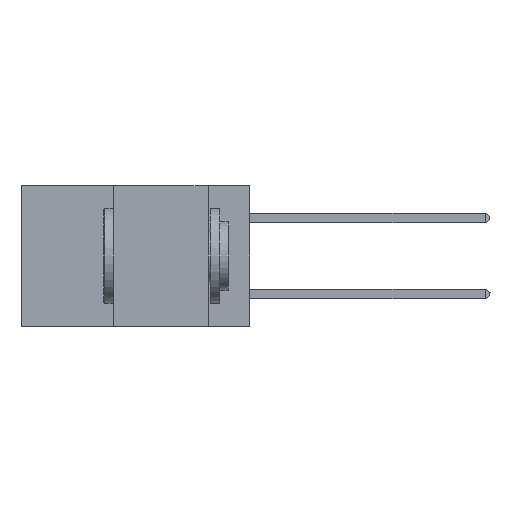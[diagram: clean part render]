
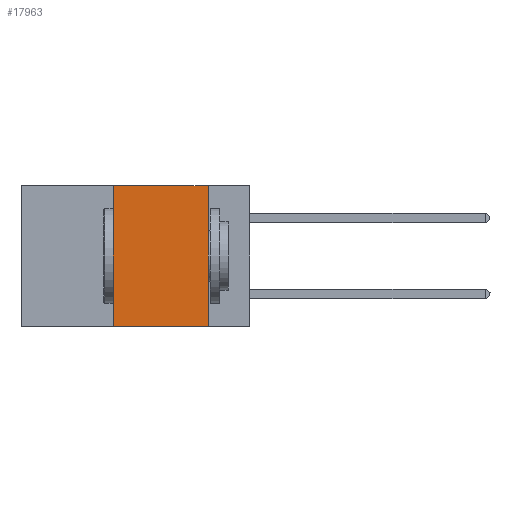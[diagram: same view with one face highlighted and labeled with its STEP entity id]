
A CAD part, left-side view. The second image highlights one B-rep face of the part: STEP entity #17963.
In plain terms, the highlighted planar face has unit normal (-1, 0, 0).
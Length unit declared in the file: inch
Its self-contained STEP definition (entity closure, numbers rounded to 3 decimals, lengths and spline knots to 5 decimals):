
#1340 = EDGE_CURVE ( 'NONE', #14689, #15010, #30542, .T. ) ;
#2039 = DIRECTION ( 'NONE',  ( 1., 0., 0. ) ) ;
#2167 = PLANE ( 'NONE',  #10971 ) ;
#4389 = CARTESIAN_POINT ( 'NONE',  ( 0., 0.6, -0.37 ) ) ;
#4546 = DIRECTION ( 'NONE',  ( 0., 0., -1. ) ) ;
#5674 = ORIENTED_EDGE ( 'NONE', *, *, #29682, .T. ) ;
#7430 = DIRECTION ( 'NONE',  ( 0., -1., 0. ) ) ;
#8201 = VECTOR ( 'NONE', #21184, 39.37008 ) ;
#9626 = EDGE_CURVE ( 'NONE', #22802, #14689, #22389, .T. ) ;
#10053 = VECTOR ( 'NONE', #22332, 39.37008 ) ;
#10971 = AXIS2_PLACEMENT_3D ( 'NONE', #28303, #2039, #33754 ) ;
#11545 = CARTESIAN_POINT ( 'NONE',  ( 0., 0.36, 0. ) ) ;
#12359 = CARTESIAN_POINT ( 'NONE',  ( 0., 0.11, -0.37 ) ) ;
#12407 = CARTESIAN_POINT ( 'NONE',  ( 0., 0.36, 0. ) ) ;
#14689 = VERTEX_POINT ( 'NONE', #24338 ) ;
#15010 = VERTEX_POINT ( 'NONE', #12359 ) ;
#16904 = FACE_OUTER_BOUND ( 'NONE', #22235, .T. ) ;
#17963 = ADVANCED_FACE ( 'NONE', ( #16904 ), #2167, .F. ) ;
#20954 = LINE ( 'NONE', #12407, #8201 ) ;
#21098 = ORIENTED_EDGE ( 'NONE', *, *, #34590, .F. ) ;
#21184 = DIRECTION ( 'NONE',  ( 0., 0., 1. ) ) ;
#22235 = EDGE_LOOP ( 'NONE', ( #29823, #26436, #21098, #5674 ) ) ;
#22261 = CARTESIAN_POINT ( 'NONE',  ( 0., 0.11, 0. ) ) ;
#22332 = DIRECTION ( 'NONE',  ( 0., -1., 0. ) ) ;
#22389 = LINE ( 'NONE', #26980, #10053 ) ;
#22802 = VERTEX_POINT ( 'NONE', #11545 ) ;
#24338 = CARTESIAN_POINT ( 'NONE',  ( 0., 0.11, 0. ) ) ;
#26038 = VECTOR ( 'NONE', #4546, 39.37008 ) ;
#26436 = ORIENTED_EDGE ( 'NONE', *, *, #9626, .F. ) ;
#26980 = CARTESIAN_POINT ( 'NONE',  ( 0., 0.6, 0. ) ) ;
#28303 = CARTESIAN_POINT ( 'NONE',  ( 0., 0.6, 0. ) ) ;
#29278 = CARTESIAN_POINT ( 'NONE',  ( 0., 0.36, -0.37 ) ) ;
#29485 = LINE ( 'NONE', #4389, #37653 ) ;
#29496 = VERTEX_POINT ( 'NONE', #29278 ) ;
#29682 = EDGE_CURVE ( 'NONE', #29496, #15010, #29485, .T. ) ;
#29823 = ORIENTED_EDGE ( 'NONE', *, *, #1340, .F. ) ;
#30542 = LINE ( 'NONE', #22261, #26038 ) ;
#33754 = DIRECTION ( 'NONE',  ( 0., 0., -1. ) ) ;
#34590 = EDGE_CURVE ( 'NONE', #29496, #22802, #20954, .T. ) ;
#37653 = VECTOR ( 'NONE', #7430, 39.37008 ) ;
